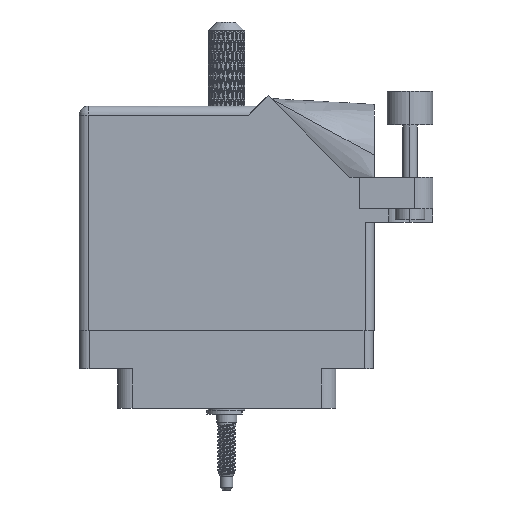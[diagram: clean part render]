
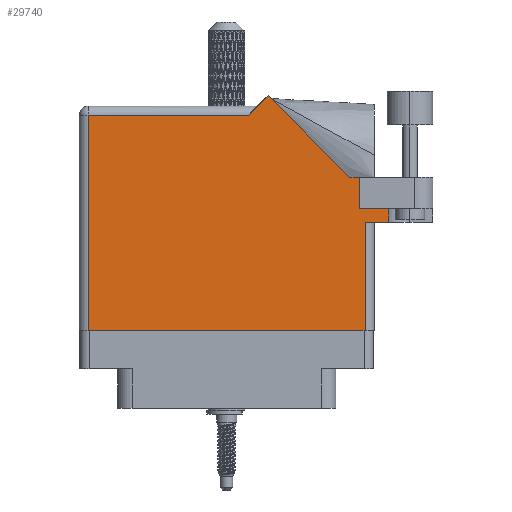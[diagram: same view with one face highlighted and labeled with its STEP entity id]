
A CAD part, front view. The second image highlights one B-rep face of the part: STEP entity #29740.
In plain terms, the highlighted face is planar.
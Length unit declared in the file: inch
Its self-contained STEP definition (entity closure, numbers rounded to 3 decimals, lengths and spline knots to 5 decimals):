
#3092 = CARTESIAN_POINT ( 'NONE',  ( 1.155, 1.468, 0. ) ) ;
#3624 = CARTESIAN_POINT ( 'NONE',  ( 1.948, 0.737, 0. ) ) ;
#3955 = CARTESIAN_POINT ( 'NONE',  ( 2.1115, 1.16177, 0. ) ) ;
#4160 = ORIENTED_EDGE ( 'NONE', *, *, #10986, .T. ) ;
#8128 = VECTOR ( 'NONE', #63003, 39.37008 ) ;
#8198 = VERTEX_POINT ( 'NONE', #52491 ) ;
#10986 = EDGE_CURVE ( 'NONE', #23539, #85162, #91895, .T. ) ;
#12806 = AXIS2_PLACEMENT_3D ( 'NONE', #103428, #53537, #13057 ) ;
#13057 = DIRECTION ( 'NONE',  ( -1., 0., 0. ) ) ;
#13147 = LINE ( 'NONE', #104969, #23350 ) ;
#14301 = LINE ( 'NONE', #81876, #79036 ) ;
#15426 = ORIENTED_EDGE ( 'NONE', *, *, #81441, .T. ) ;
#15458 = ORIENTED_EDGE ( 'NONE', *, *, #100931, .T. ) ;
#16012 = ORIENTED_EDGE ( 'NONE', *, *, #30940, .T. ) ;
#16710 = CARTESIAN_POINT ( 'NONE',  ( 1.28771, 1.60071, 0. ) ) ;
#18206 = VERTEX_POINT ( 'NONE', #81098 ) ;
#20715 = DIRECTION ( 'NONE',  ( 0., -1., 0. ) ) ;
#23350 = VECTOR ( 'NONE', #96807, 39.37008 ) ;
#23377 = ORIENTED_EDGE ( 'NONE', *, *, #53844, .T. ) ;
#23539 = VERTEX_POINT ( 'NONE', #62085 ) ;
#24358 = LINE ( 'NONE', #76435, #92833 ) ;
#27126 = FACE_OUTER_BOUND ( 'NONE', #86510, .T. ) ;
#27703 = VECTOR ( 'NONE', #84483, 39.37008 ) ;
#28156 = CARTESIAN_POINT ( 'NONE',  ( 1.91, 0.831, 0. ) ) ;
#29196 = EDGE_CURVE ( 'NONE', #36692, #55303, #46349, .T. ) ;
#29740 = ADVANCED_FACE ( 'NONE', ( #27126 ), #93881, .F. ) ;
#30251 = VERTEX_POINT ( 'NONE', #3624 ) ;
#30940 = EDGE_CURVE ( 'NONE', #8198, #18206, #14301, .T. ) ;
#34579 = ORIENTED_EDGE ( 'NONE', *, *, #29196, .T. ) ;
#34862 = EDGE_CURVE ( 'NONE', #23539, #86782, #96196, .T. ) ;
#35662 = LINE ( 'NONE', #59119, #81298 ) ;
#35990 = LINE ( 'NONE', #79581, #55030 ) ;
#36692 = VERTEX_POINT ( 'NONE', #16710 ) ;
#42550 = LINE ( 'NONE', #55928, #8128 ) ;
#43520 = VERTEX_POINT ( 'NONE', #95187 ) ;
#46349 = LINE ( 'NONE', #66095, #98172 ) ;
#48083 = DIRECTION ( 'NONE',  ( 0., -1., 0. ) ) ;
#48816 = VECTOR ( 'NONE', #76780, 39.37008 ) ;
#51523 = EDGE_CURVE ( 'NONE', #86782, #100276, #76294, .T. ) ;
#52491 = CARTESIAN_POINT ( 'NONE',  ( 0.062, 0., 0. ) ) ;
#53537 = DIRECTION ( 'NONE',  ( 0., 0., -1. ) ) ;
#53844 = EDGE_CURVE ( 'NONE', #60901, #36692, #64560, .T. ) ;
#55030 = VECTOR ( 'NONE', #48083, 39.37008 ) ;
#55303 = VERTEX_POINT ( 'NONE', #3092 ) ;
#55928 = CARTESIAN_POINT ( 'NONE',  ( 2.41, 1.044, 0. ) ) ;
#59119 = CARTESIAN_POINT ( 'NONE',  ( 2.01, 0.737, 0. ) ) ;
#60901 = VERTEX_POINT ( 'NONE', #100229 ) ;
#61064 = EDGE_CURVE ( 'NONE', #85162, #60901, #42550, .T. ) ;
#62085 = CARTESIAN_POINT ( 'NONE',  ( 1.91, 0.831, 0. ) ) ;
#63003 = DIRECTION ( 'NONE',  ( -1., 0., 0. ) ) ;
#64560 = LINE ( 'NONE', #85197, #27703 ) ;
#66095 = CARTESIAN_POINT ( 'NONE',  ( 1.217, 1.53, 0. ) ) ;
#68533 = EDGE_CURVE ( 'NONE', #43520, #8198, #35990, .T. ) ;
#70485 = CARTESIAN_POINT ( 'NONE',  ( 2.1115, 0.737, 0. ) ) ;
#76294 = LINE ( 'NONE', #3955, #82671 ) ;
#76435 = CARTESIAN_POINT ( 'NONE',  ( 1.948, 0.737, 0. ) ) ;
#76780 = DIRECTION ( 'NONE',  ( 0., 1., 0. ) ) ;
#76893 = CARTESIAN_POINT ( 'NONE',  ( 1.91, 1.044, 0. ) ) ;
#77156 = DIRECTION ( 'NONE',  ( 1., 0., 0. ) ) ;
#79036 = VECTOR ( 'NONE', #90722, 39.37008 ) ;
#79581 = CARTESIAN_POINT ( 'NONE',  ( 0.062, 0., 0. ) ) ;
#80624 = DIRECTION ( 'NONE',  ( -0.707, -0.707, 0. ) ) ;
#81098 = CARTESIAN_POINT ( 'NONE',  ( 1.948, 0., 0. ) ) ;
#81298 = VECTOR ( 'NONE', #100539, 39.37008 ) ;
#81441 = EDGE_CURVE ( 'NONE', #18206, #30251, #24358, .T. ) ;
#81876 = CARTESIAN_POINT ( 'NONE',  ( 0., 0., 0. ) ) ;
#82671 = VECTOR ( 'NONE', #20715, 39.37008 ) ;
#82865 = ORIENTED_EDGE ( 'NONE', *, *, #68533, .T. ) ;
#84472 = ORIENTED_EDGE ( 'NONE', *, *, #34862, .F. ) ;
#84483 = DIRECTION ( 'NONE',  ( -0.707, 0.707, 0. ) ) ;
#85162 = VERTEX_POINT ( 'NONE', #76893 ) ;
#85197 = CARTESIAN_POINT ( 'NONE',  ( 1.84442, 1.044, 0. ) ) ;
#86510 = EDGE_LOOP ( 'NONE', ( #16012, #15426, #15458, #96794, #84472, #4160, #97892, #23377, #34579, #89046, #82865 ) ) ;
#86782 = VERTEX_POINT ( 'NONE', #98776 ) ;
#89046 = ORIENTED_EDGE ( 'NONE', *, *, #89635, .T. ) ;
#89635 = EDGE_CURVE ( 'NONE', #55303, #43520, #13147, .T. ) ;
#90722 = DIRECTION ( 'NONE',  ( 1., 0., 0. ) ) ;
#91895 = LINE ( 'NONE', #28156, #48816 ) ;
#92687 = DIRECTION ( 'NONE',  ( 0., 1., 0. ) ) ;
#92833 = VECTOR ( 'NONE', #92687, 39.37008 ) ;
#93881 = PLANE ( 'NONE',  #12806 ) ;
#95187 = CARTESIAN_POINT ( 'NONE',  ( 0.062, 1.468, 0. ) ) ;
#96196 = LINE ( 'NONE', #101556, #98700 ) ;
#96794 = ORIENTED_EDGE ( 'NONE', *, *, #51523, .F. ) ;
#96807 = DIRECTION ( 'NONE',  ( -1., 0., 0. ) ) ;
#97892 = ORIENTED_EDGE ( 'NONE', *, *, #61064, .T. ) ;
#98172 = VECTOR ( 'NONE', #80624, 39.37008 ) ;
#98700 = VECTOR ( 'NONE', #77156, 39.37008 ) ;
#98776 = CARTESIAN_POINT ( 'NONE',  ( 2.1115, 0.831, 0. ) ) ;
#100229 = CARTESIAN_POINT ( 'NONE',  ( 1.84442, 1.044, 0. ) ) ;
#100276 = VERTEX_POINT ( 'NONE', #70485 ) ;
#100539 = DIRECTION ( 'NONE',  ( 1., 0., 0. ) ) ;
#100931 = EDGE_CURVE ( 'NONE', #30251, #100276, #35662, .T. ) ;
#101556 = CARTESIAN_POINT ( 'NONE',  ( 1.91, 0.831, 0. ) ) ;
#103428 = CARTESIAN_POINT ( 'NONE',  ( 0., 1.53, 0. ) ) ;
#104969 = CARTESIAN_POINT ( 'NONE',  ( 0., 1.468, 0. ) ) ;
